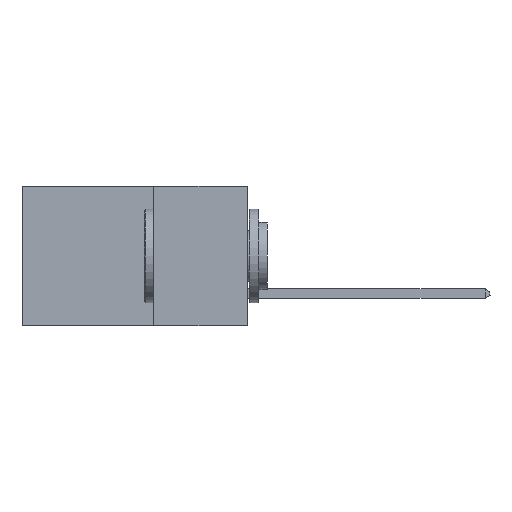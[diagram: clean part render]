
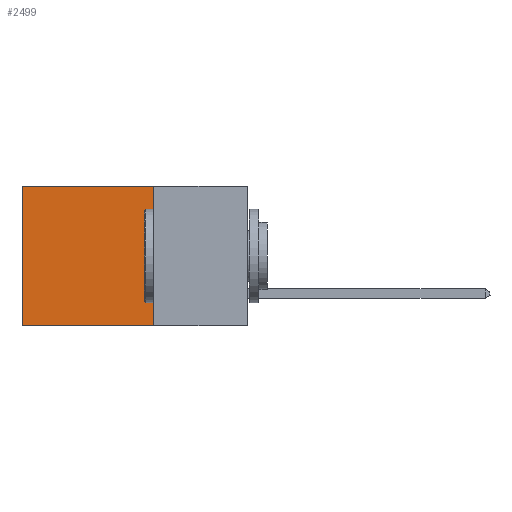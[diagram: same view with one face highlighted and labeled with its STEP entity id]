
A CAD part, left-side view. The second image highlights one B-rep face of the part: STEP entity #2499.
In plain terms, the highlighted planar face has unit normal (-1, 0, 0).
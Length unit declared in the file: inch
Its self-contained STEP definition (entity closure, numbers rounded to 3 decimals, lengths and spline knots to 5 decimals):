
#88 = VECTOR ( 'NONE', #7013, 39.37008 ) ;
#683 = VECTOR ( 'NONE', #10804, 39.37008 ) ;
#1271 = ORIENTED_EDGE ( 'NONE', *, *, #8091, .T. ) ;
#1528 = CARTESIAN_POINT ( 'NONE',  ( 0.298, 0.25, -0.37 ) ) ;
#1751 = VECTOR ( 'NONE', #6578, 39.37008 ) ;
#1838 = ORIENTED_EDGE ( 'NONE', *, *, #4280, .F. ) ;
#2499 = ADVANCED_FACE ( 'NONE', ( #9679 ), #9757, .F. ) ;
#2850 = CARTESIAN_POINT ( 'NONE',  ( 0.298, 0.25, 0. ) ) ;
#3024 = VECTOR ( 'NONE', #12480, 39.37008 ) ;
#3278 = LINE ( 'NONE', #4375, #683 ) ;
#4280 = EDGE_CURVE ( 'NONE', #10148, #7250, #10975, .T. ) ;
#4375 = CARTESIAN_POINT ( 'NONE',  ( 0.298, 0.25, 0. ) ) ;
#5923 = CARTESIAN_POINT ( 'NONE',  ( 0.298, 0.25, 0. ) ) ;
#6268 = VERTEX_POINT ( 'NONE', #6603 ) ;
#6578 = DIRECTION ( 'NONE',  ( 0., 1., 0. ) ) ;
#6603 = CARTESIAN_POINT ( 'NONE',  ( 0.298, 0.6, -0.37 ) ) ;
#7013 = DIRECTION ( 'NONE',  ( 0., 0., -1. ) ) ;
#7250 = VERTEX_POINT ( 'NONE', #15601 ) ;
#7320 = CARTESIAN_POINT ( 'NONE',  ( 0.298, 0.25, 0. ) ) ;
#7628 = VERTEX_POINT ( 'NONE', #13870 ) ;
#8091 = EDGE_CURVE ( 'NONE', #7628, #6268, #10843, .T. ) ;
#8372 = EDGE_CURVE ( 'NONE', #10148, #7628, #3278, .T. ) ;
#8736 = AXIS2_PLACEMENT_3D ( 'NONE', #5923, #9654, #12376 ) ;
#9563 = CARTESIAN_POINT ( 'NONE',  ( 0.298, 0.6, 0. ) ) ;
#9654 = DIRECTION ( 'NONE',  ( 1., 0., 0. ) ) ;
#9679 = FACE_OUTER_BOUND ( 'NONE', #9944, .T. ) ;
#9757 = PLANE ( 'NONE',  #8736 ) ;
#9944 = EDGE_LOOP ( 'NONE', ( #1271, #12869, #1838, #13961 ) ) ;
#10077 = EDGE_CURVE ( 'NONE', #7250, #6268, #11077, .T. ) ;
#10148 = VERTEX_POINT ( 'NONE', #2850 ) ;
#10804 = DIRECTION ( 'NONE',  ( 0., 1., 0. ) ) ;
#10843 = LINE ( 'NONE', #9563, #88 ) ;
#10975 = LINE ( 'NONE', #7320, #3024 ) ;
#11077 = LINE ( 'NONE', #1528, #1751 ) ;
#12376 = DIRECTION ( 'NONE',  ( 0., 0., -1. ) ) ;
#12480 = DIRECTION ( 'NONE',  ( 0., 0., -1. ) ) ;
#12869 = ORIENTED_EDGE ( 'NONE', *, *, #10077, .F. ) ;
#13870 = CARTESIAN_POINT ( 'NONE',  ( 0.298, 0.6, 0. ) ) ;
#13961 = ORIENTED_EDGE ( 'NONE', *, *, #8372, .T. ) ;
#15601 = CARTESIAN_POINT ( 'NONE',  ( 0.298, 0.25, -0.37 ) ) ;
